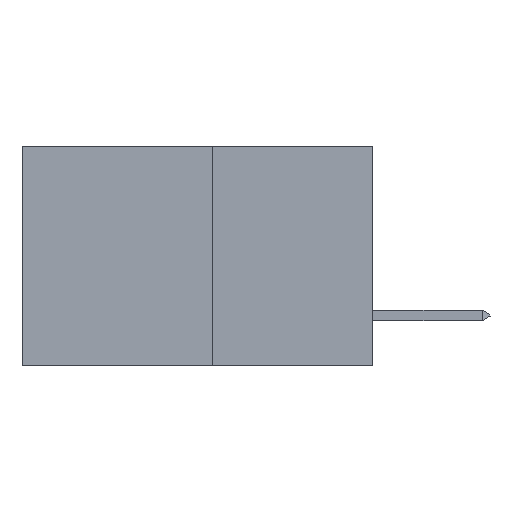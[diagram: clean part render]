
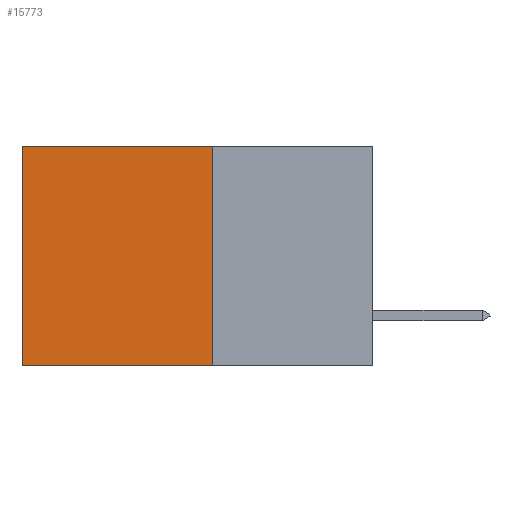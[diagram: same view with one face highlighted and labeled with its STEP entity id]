
A CAD part, left-side view. The second image highlights one B-rep face of the part: STEP entity #15773.
In plain terms, the highlighted planar face has unit normal (-1, 0, 0).
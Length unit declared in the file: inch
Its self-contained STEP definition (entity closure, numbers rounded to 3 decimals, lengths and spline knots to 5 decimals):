
#1503 = FACE_OUTER_BOUND ( 'NONE', #12812, .T. ) ;
#1868 = EDGE_CURVE ( 'NONE', #10505, #11734, #22060, .T. ) ;
#2677 = DIRECTION ( 'NONE',  ( 1., 0., 0. ) ) ;
#4385 = LINE ( 'NONE', #11550, #15232 ) ;
#4891 = VECTOR ( 'NONE', #10135, 39.37008 ) ;
#5087 = ORIENTED_EDGE ( 'NONE', *, *, #12363, .F. ) ;
#5821 = CARTESIAN_POINT ( 'NONE',  ( 0.277, 0.27, 0. ) ) ;
#9162 = CARTESIAN_POINT ( 'NONE',  ( 0.277, 0.27, -0.37 ) ) ;
#9715 = ORIENTED_EDGE ( 'NONE', *, *, #24320, .T. ) ;
#10135 = DIRECTION ( 'NONE',  ( 0., 1., 0. ) ) ;
#10505 = VERTEX_POINT ( 'NONE', #20264 ) ;
#11319 = VERTEX_POINT ( 'NONE', #5821 ) ;
#11369 = VECTOR ( 'NONE', #12542, 39.37008 ) ;
#11550 = CARTESIAN_POINT ( 'NONE',  ( 0.277, 0.27, -0.37 ) ) ;
#11661 = CARTESIAN_POINT ( 'NONE',  ( 0.277, 0.27, -0.37 ) ) ;
#11734 = VERTEX_POINT ( 'NONE', #24299 ) ;
#12176 = ORIENTED_EDGE ( 'NONE', *, *, #15590, .T. ) ;
#12363 = EDGE_CURVE ( 'NONE', #11319, #10505, #4385, .T. ) ;
#12542 = DIRECTION ( 'NONE',  ( 0., 1., 0. ) ) ;
#12812 = EDGE_LOOP ( 'NONE', ( #9715, #25144, #5087, #12176 ) ) ;
#13315 = VECTOR ( 'NONE', #17636, 39.37008 ) ;
#13716 = DIRECTION ( 'NONE',  ( 0., 0., -1. ) ) ;
#14616 = CARTESIAN_POINT ( 'NONE',  ( 0.277, 0.27, 0. ) ) ;
#15232 = VECTOR ( 'NONE', #13716, 39.37008 ) ;
#15484 = CARTESIAN_POINT ( 'NONE',  ( 0.277, 0.59, -0.37 ) ) ;
#15590 = EDGE_CURVE ( 'NONE', #11319, #22671, #17759, .T. ) ;
#15773 = ADVANCED_FACE ( 'NONE', ( #1503 ), #19481, .F. ) ;
#17636 = DIRECTION ( 'NONE',  ( 0., 0., -1. ) ) ;
#17759 = LINE ( 'NONE', #14616, #11369 ) ;
#17806 = DIRECTION ( 'NONE',  ( 0., 0., -1. ) ) ;
#19341 = AXIS2_PLACEMENT_3D ( 'NONE', #9162, #2677, #17806 ) ;
#19481 = PLANE ( 'NONE',  #19341 ) ;
#19691 = LINE ( 'NONE', #15484, #13315 ) ;
#20264 = CARTESIAN_POINT ( 'NONE',  ( 0.277, 0.27, -0.37 ) ) ;
#20324 = CARTESIAN_POINT ( 'NONE',  ( 0.277, 0.59, 0. ) ) ;
#22060 = LINE ( 'NONE', #11661, #4891 ) ;
#22671 = VERTEX_POINT ( 'NONE', #20324 ) ;
#24299 = CARTESIAN_POINT ( 'NONE',  ( 0.277, 0.59, -0.37 ) ) ;
#24320 = EDGE_CURVE ( 'NONE', #22671, #11734, #19691, .T. ) ;
#25144 = ORIENTED_EDGE ( 'NONE', *, *, #1868, .F. ) ;
